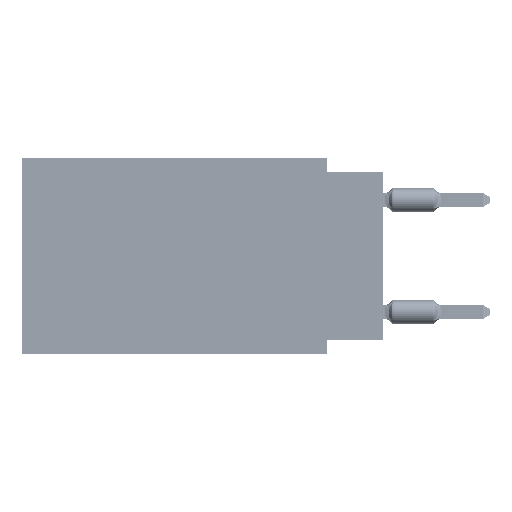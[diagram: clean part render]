
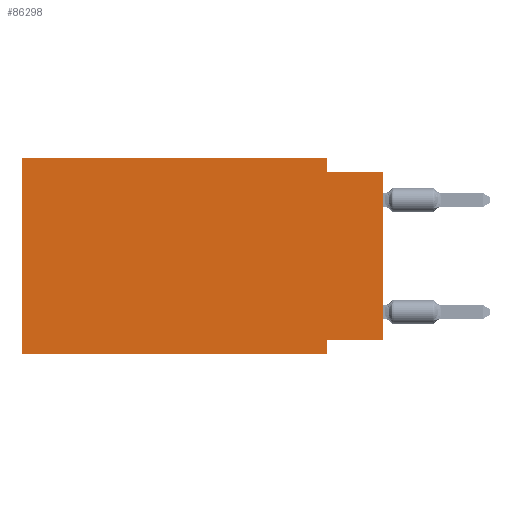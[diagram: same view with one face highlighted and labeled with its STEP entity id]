
A CAD part, left-side view. The second image highlights one B-rep face of the part: STEP entity #86298.
In plain terms, the highlighted planar face has unit normal (-1, 0, 0).
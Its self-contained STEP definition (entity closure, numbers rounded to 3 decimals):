
#1990 = VECTOR ( 'NONE', #98450, 1000. ) ;
#2049 = PLANE ( 'NONE',  #13031 ) ;
#2251 = CARTESIAN_POINT ( 'NONE',  ( 0., 2.54, 0. ) ) ;
#3017 = CARTESIAN_POINT ( 'NONE',  ( 0., 16.383, 0. ) ) ;
#3140 = CARTESIAN_POINT ( 'NONE',  ( 0., 16.383, -8.89 ) ) ;
#3187 = CARTESIAN_POINT ( 'NONE',  ( 0., 2.54, -8.255 ) ) ;
#5370 = LINE ( 'NONE', #39106, #36678 ) ;
#5761 = VECTOR ( 'NONE', #35562, 1000. ) ;
#6028 = LINE ( 'NONE', #48622, #44863 ) ;
#6363 = VERTEX_POINT ( 'NONE', #58694 ) ;
#9255 = FACE_OUTER_BOUND ( 'NONE', #108208, .T. ) ;
#9969 = ORIENTED_EDGE ( 'NONE', *, *, #101808, .F. ) ;
#11445 = DIRECTION ( 'NONE',  ( 0., 0., -1. ) ) ;
#13031 = AXIS2_PLACEMENT_3D ( 'NONE', #51840, #87237, #11445 ) ;
#13890 = VECTOR ( 'NONE', #103174, 1000. ) ;
#14908 = CARTESIAN_POINT ( 'NONE',  ( 0., 16.383, 0. ) ) ;
#14938 = ORIENTED_EDGE ( 'NONE', *, *, #53991, .F. ) ;
#19357 = VECTOR ( 'NONE', #40771, 1000. ) ;
#23625 = LINE ( 'NONE', #47969, #19357 ) ;
#23917 = CARTESIAN_POINT ( 'NONE',  ( 0., 2.54, -8.89 ) ) ;
#25381 = EDGE_CURVE ( 'NONE', #67618, #39710, #46141, .T. ) ;
#25572 = DIRECTION ( 'NONE',  ( 0., 1., 0. ) ) ;
#29336 = ORIENTED_EDGE ( 'NONE', *, *, #98789, .T. ) ;
#31746 = CARTESIAN_POINT ( 'NONE',  ( 0., 0., 0. ) ) ;
#31973 = VERTEX_POINT ( 'NONE', #3187 ) ;
#33539 = VERTEX_POINT ( 'NONE', #66127 ) ;
#35562 = DIRECTION ( 'NONE',  ( 0., 0., 1. ) ) ;
#36678 = VECTOR ( 'NONE', #106635, 1000. ) ;
#36869 = DIRECTION ( 'NONE',  ( 0., -1., 0. ) ) ;
#37058 = ORIENTED_EDGE ( 'NONE', *, *, #66950, .T. ) ;
#38128 = EDGE_CURVE ( 'NONE', #39710, #33539, #6028, .T. ) ;
#39106 = CARTESIAN_POINT ( 'NONE',  ( 0., 0., -0.635 ) ) ;
#39710 = VERTEX_POINT ( 'NONE', #2251 ) ;
#39812 = LINE ( 'NONE', #14908, #1990 ) ;
#40771 = DIRECTION ( 'NONE',  ( 0., 0., -1. ) ) ;
#43692 = CARTESIAN_POINT ( 'NONE',  ( 0., 16.383, 0. ) ) ;
#44863 = VECTOR ( 'NONE', #49707, 1000. ) ;
#45722 = LINE ( 'NONE', #3140, #95088 ) ;
#46141 = LINE ( 'NONE', #3017, #13890 ) ;
#46235 = ORIENTED_EDGE ( 'NONE', *, *, #77591, .F. ) ;
#47969 = CARTESIAN_POINT ( 'NONE',  ( 0., 2.54, -8.89 ) ) ;
#48622 = CARTESIAN_POINT ( 'NONE',  ( 0., 2.54, 0. ) ) ;
#49707 = DIRECTION ( 'NONE',  ( 0., 0., -1. ) ) ;
#51840 = CARTESIAN_POINT ( 'NONE',  ( 0., 16.383, 0. ) ) ;
#53991 = EDGE_CURVE ( 'NONE', #71836, #31973, #67048, .T. ) ;
#56698 = VERTEX_POINT ( 'NONE', #23917 ) ;
#58694 = CARTESIAN_POINT ( 'NONE',  ( 0., 16.383, -8.89 ) ) ;
#62844 = ORIENTED_EDGE ( 'NONE', *, *, #38128, .F. ) ;
#66127 = CARTESIAN_POINT ( 'NONE',  ( 0., 2.54, -0.635 ) ) ;
#66950 = EDGE_CURVE ( 'NONE', #6363, #56698, #45722, .T. ) ;
#67048 = LINE ( 'NONE', #92524, #74634 ) ;
#67618 = VERTEX_POINT ( 'NONE', #43692 ) ;
#71836 = VERTEX_POINT ( 'NONE', #96708 ) ;
#74634 = VECTOR ( 'NONE', #25572, 1000. ) ;
#77591 = EDGE_CURVE ( 'NONE', #33539, #82461, #5370, .T. ) ;
#81737 = ORIENTED_EDGE ( 'NONE', *, *, #83339, .F. ) ;
#82120 = LINE ( 'NONE', #31746, #5761 ) ;
#82461 = VERTEX_POINT ( 'NONE', #104849 ) ;
#83339 = EDGE_CURVE ( 'NONE', #6363, #67618, #39812, .T. ) ;
#86298 = ADVANCED_FACE ( 'NONE', ( #9255 ), #2049, .F. ) ;
#87237 = DIRECTION ( 'NONE',  ( 1., 0., 0. ) ) ;
#92524 = CARTESIAN_POINT ( 'NONE',  ( 0., 0., -8.255 ) ) ;
#95088 = VECTOR ( 'NONE', #36869, 1000. ) ;
#96708 = CARTESIAN_POINT ( 'NONE',  ( 0., 0., -8.255 ) ) ;
#98450 = DIRECTION ( 'NONE',  ( 0., 0., 1. ) ) ;
#98789 = EDGE_CURVE ( 'NONE', #71836, #82461, #82120, .T. ) ;
#101808 = EDGE_CURVE ( 'NONE', #31973, #56698, #23625, .T. ) ;
#103174 = DIRECTION ( 'NONE',  ( 0., -1., 0. ) ) ;
#104849 = CARTESIAN_POINT ( 'NONE',  ( 0., 0., -0.635 ) ) ;
#106287 = ORIENTED_EDGE ( 'NONE', *, *, #25381, .F. ) ;
#106635 = DIRECTION ( 'NONE',  ( 0., -1., 0. ) ) ;
#108208 = EDGE_LOOP ( 'NONE', ( #29336, #46235, #62844, #106287, #81737, #37058, #9969, #14938 ) ) ;
